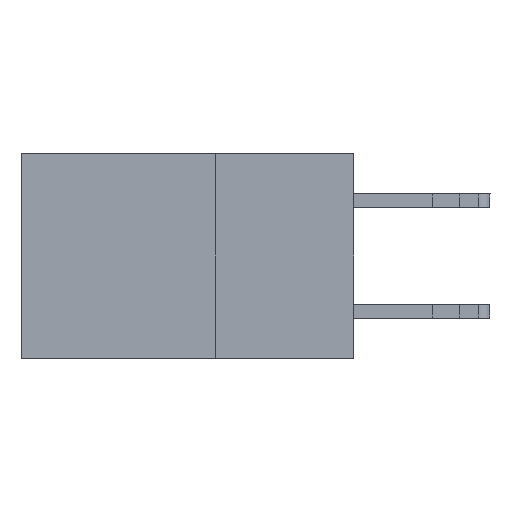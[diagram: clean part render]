
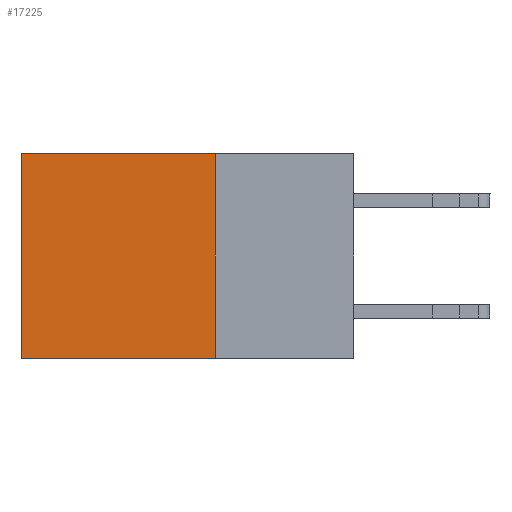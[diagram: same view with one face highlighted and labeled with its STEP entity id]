
A CAD part, left-side view. The second image highlights one B-rep face of the part: STEP entity #17225.
In plain terms, the highlighted planar face has unit normal (-1, 0, 0).
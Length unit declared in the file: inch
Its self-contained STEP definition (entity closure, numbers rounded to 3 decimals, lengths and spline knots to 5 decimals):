
#33 = ORIENTED_EDGE ( 'NONE', *, *, #13534, .T. ) ;
#414 = DIRECTION ( 'NONE',  ( 0., 0., -1. ) ) ;
#1521 = VERTEX_POINT ( 'NONE', #16084 ) ;
#1578 = CARTESIAN_POINT ( 'NONE',  ( 0.2875, 0.25, 0. ) ) ;
#2123 = VECTOR ( 'NONE', #24324, 39.37008 ) ;
#3340 = ORIENTED_EDGE ( 'NONE', *, *, #9315, .T. ) ;
#3803 = CARTESIAN_POINT ( 'NONE',  ( 0.2875, 0.25, 0. ) ) ;
#3813 = VERTEX_POINT ( 'NONE', #6096 ) ;
#4690 = CARTESIAN_POINT ( 'NONE',  ( 0.2875, 0.6, 0. ) ) ;
#5212 = LINE ( 'NONE', #1578, #21661 ) ;
#5484 = AXIS2_PLACEMENT_3D ( 'NONE', #3803, #11393, #9066 ) ;
#6096 = CARTESIAN_POINT ( 'NONE',  ( 0.2875, 0.6, 0. ) ) ;
#6462 = DIRECTION ( 'NONE',  ( 0., 1., 0. ) ) ;
#7206 = PLANE ( 'NONE',  #5484 ) ;
#9066 = DIRECTION ( 'NONE',  ( 0., 0., -1. ) ) ;
#9250 = CARTESIAN_POINT ( 'NONE',  ( 0.2875, 0.25, -0.37 ) ) ;
#9315 = EDGE_CURVE ( 'NONE', #3813, #1521, #20987, .T. ) ;
#11138 = EDGE_CURVE ( 'NONE', #18038, #1521, #12288, .T. ) ;
#11393 = DIRECTION ( 'NONE',  ( 1., 0., 0. ) ) ;
#12288 = LINE ( 'NONE', #20026, #21167 ) ;
#12460 = EDGE_LOOP ( 'NONE', ( #3340, #20530, #15643, #33 ) ) ;
#13534 = EDGE_CURVE ( 'NONE', #16562, #3813, #5212, .T. ) ;
#15643 = ORIENTED_EDGE ( 'NONE', *, *, #22206, .F. ) ;
#16084 = CARTESIAN_POINT ( 'NONE',  ( 0.2875, 0.6, -0.37 ) ) ;
#16562 = VERTEX_POINT ( 'NONE', #19677 ) ;
#17225 = ADVANCED_FACE ( 'NONE', ( #24302 ), #7206, .F. ) ;
#18038 = VERTEX_POINT ( 'NONE', #9250 ) ;
#18045 = VECTOR ( 'NONE', #414, 39.37008 ) ;
#19677 = CARTESIAN_POINT ( 'NONE',  ( 0.2875, 0.25, 0. ) ) ;
#20026 = CARTESIAN_POINT ( 'NONE',  ( 0.2875, 0.25, -0.37 ) ) ;
#20270 = LINE ( 'NONE', #23953, #2123 ) ;
#20530 = ORIENTED_EDGE ( 'NONE', *, *, #11138, .F. ) ;
#20987 = LINE ( 'NONE', #4690, #18045 ) ;
#21167 = VECTOR ( 'NONE', #6462, 39.37008 ) ;
#21661 = VECTOR ( 'NONE', #21842, 39.37008 ) ;
#21842 = DIRECTION ( 'NONE',  ( 0., 1., 0. ) ) ;
#22206 = EDGE_CURVE ( 'NONE', #16562, #18038, #20270, .T. ) ;
#23953 = CARTESIAN_POINT ( 'NONE',  ( 0.2875, 0.25, 0. ) ) ;
#24302 = FACE_OUTER_BOUND ( 'NONE', #12460, .T. ) ;
#24324 = DIRECTION ( 'NONE',  ( 0., 0., -1. ) ) ;
